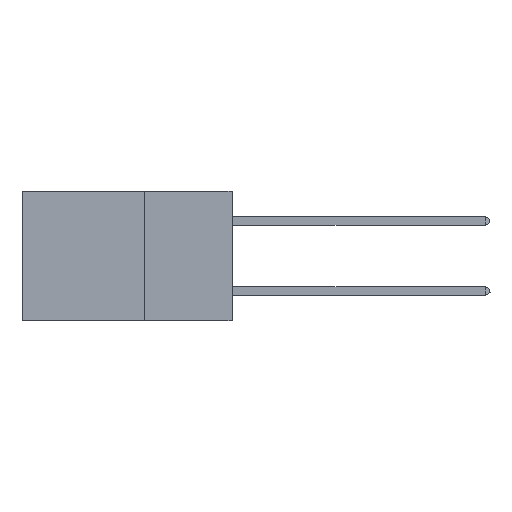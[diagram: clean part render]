
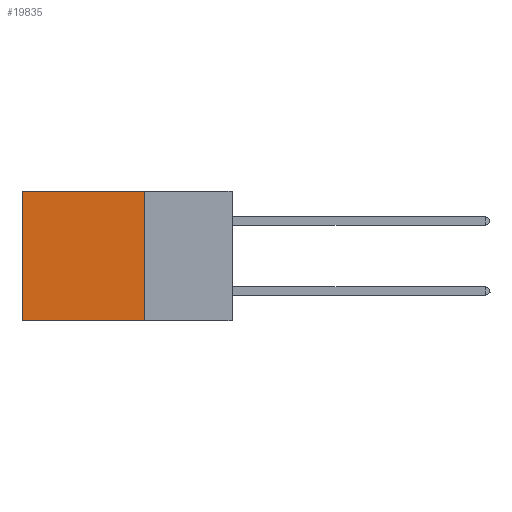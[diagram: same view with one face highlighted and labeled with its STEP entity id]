
A CAD part, left-side view. The second image highlights one B-rep face of the part: STEP entity #19835.
In plain terms, the highlighted planar face has unit normal (-1, 0, 0).
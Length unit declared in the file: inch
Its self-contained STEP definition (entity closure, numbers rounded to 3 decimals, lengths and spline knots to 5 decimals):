
#1554 = CARTESIAN_POINT ( 'NONE',  ( 0.2875, 0.25, 0. ) ) ;
#3086 = VERTEX_POINT ( 'NONE', #27348 ) ;
#5111 = LINE ( 'NONE', #14347, #16211 ) ;
#6221 = VERTEX_POINT ( 'NONE', #29307 ) ;
#6650 = ORIENTED_EDGE ( 'NONE', *, *, #26180, .T. ) ;
#6948 = ORIENTED_EDGE ( 'NONE', *, *, #33586, .T. ) ;
#7416 = EDGE_CURVE ( 'NONE', #16769, #6221, #29815, .T. ) ;
#8998 = LINE ( 'NONE', #22871, #24811 ) ;
#10220 = AXIS2_PLACEMENT_3D ( 'NONE', #1554, #34559, #15512 ) ;
#13016 = LINE ( 'NONE', #33977, #19388 ) ;
#14347 = CARTESIAN_POINT ( 'NONE',  ( 0.2875, 0.25, 0. ) ) ;
#15512 = DIRECTION ( 'NONE',  ( 0., 0., -1. ) ) ;
#16211 = VECTOR ( 'NONE', #23388, 39.37008 ) ;
#16769 = VERTEX_POINT ( 'NONE', #24931 ) ;
#19110 = EDGE_CURVE ( 'NONE', #3086, #16769, #5111, .T. ) ;
#19388 = VECTOR ( 'NONE', #31099, 39.37008 ) ;
#19593 = DIRECTION ( 'NONE',  ( 0., 1., 0. ) ) ;
#19835 = ADVANCED_FACE ( 'NONE', ( #31122 ), #34439, .F. ) ;
#22227 = ORIENTED_EDGE ( 'NONE', *, *, #19110, .F. ) ;
#22480 = EDGE_LOOP ( 'NONE', ( #6948, #31790, #22227, #6650 ) ) ;
#22575 = CARTESIAN_POINT ( 'NONE',  ( 0.2875, 0.25, -0.37 ) ) ;
#22871 = CARTESIAN_POINT ( 'NONE',  ( 0.2875, 0.25, 0. ) ) ;
#22931 = VECTOR ( 'NONE', #19593, 39.37008 ) ;
#23388 = DIRECTION ( 'NONE',  ( 0., 0., -1. ) ) ;
#24811 = VECTOR ( 'NONE', #28084, 39.37008 ) ;
#24931 = CARTESIAN_POINT ( 'NONE',  ( 0.2875, 0.25, -0.37 ) ) ;
#26180 = EDGE_CURVE ( 'NONE', #3086, #27834, #8998, .T. ) ;
#27348 = CARTESIAN_POINT ( 'NONE',  ( 0.2875, 0.25, 0. ) ) ;
#27834 = VERTEX_POINT ( 'NONE', #31540 ) ;
#28084 = DIRECTION ( 'NONE',  ( 0., 1., 0. ) ) ;
#29307 = CARTESIAN_POINT ( 'NONE',  ( 0.2875, 0.6, -0.37 ) ) ;
#29815 = LINE ( 'NONE', #22575, #22931 ) ;
#31099 = DIRECTION ( 'NONE',  ( 0., 0., -1. ) ) ;
#31122 = FACE_OUTER_BOUND ( 'NONE', #22480, .T. ) ;
#31540 = CARTESIAN_POINT ( 'NONE',  ( 0.2875, 0.6, 0. ) ) ;
#31790 = ORIENTED_EDGE ( 'NONE', *, *, #7416, .F. ) ;
#33586 = EDGE_CURVE ( 'NONE', #27834, #6221, #13016, .T. ) ;
#33977 = CARTESIAN_POINT ( 'NONE',  ( 0.2875, 0.6, 0. ) ) ;
#34439 = PLANE ( 'NONE',  #10220 ) ;
#34559 = DIRECTION ( 'NONE',  ( 1., 0., 0. ) ) ;
